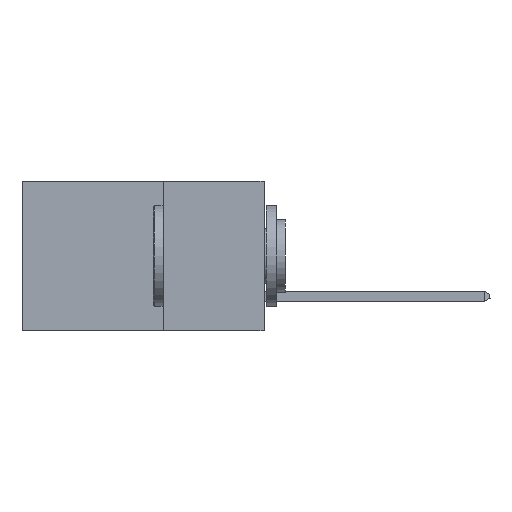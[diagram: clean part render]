
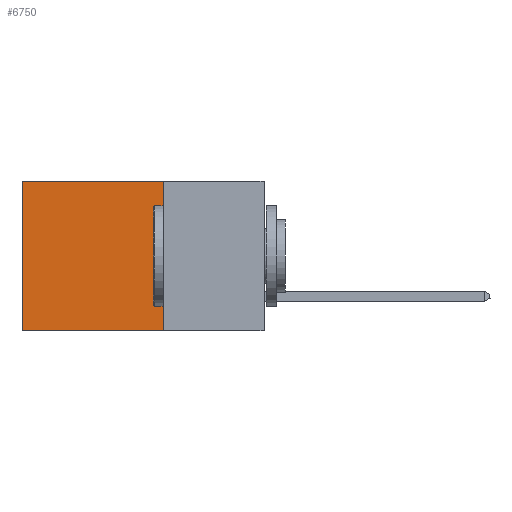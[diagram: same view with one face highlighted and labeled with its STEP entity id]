
A CAD part, left-side view. The second image highlights one B-rep face of the part: STEP entity #6750.
In plain terms, the highlighted planar face has unit normal (-1, 0, 0).
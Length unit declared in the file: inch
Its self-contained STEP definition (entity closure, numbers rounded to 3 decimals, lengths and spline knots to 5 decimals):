
#143 = VERTEX_POINT ( 'NONE', #7188 ) ;
#413 = CARTESIAN_POINT ( 'NONE',  ( 0.298, 0.6, 0. ) ) ;
#593 = LINE ( 'NONE', #413, #1870 ) ;
#605 = VERTEX_POINT ( 'NONE', #2450 ) ;
#1080 = VECTOR ( 'NONE', #4341, 39.37008 ) ;
#1273 = DIRECTION ( 'NONE',  ( 0., 0., -1. ) ) ;
#1441 = VECTOR ( 'NONE', #8896, 39.37008 ) ;
#1870 = VECTOR ( 'NONE', #4337, 39.37008 ) ;
#2033 = CARTESIAN_POINT ( 'NONE',  ( 0.298, 0.25, 0. ) ) ;
#2450 = CARTESIAN_POINT ( 'NONE',  ( 0.298, 0.6, -0.37 ) ) ;
#2784 = CARTESIAN_POINT ( 'NONE',  ( 0.298, 0.25, 0. ) ) ;
#2897 = EDGE_CURVE ( 'NONE', #7381, #605, #6038, .T. ) ;
#3530 = FACE_OUTER_BOUND ( 'NONE', #5600, .T. ) ;
#4065 = VECTOR ( 'NONE', #9885, 39.37008 ) ;
#4132 = LINE ( 'NONE', #2784, #1080 ) ;
#4238 = ORIENTED_EDGE ( 'NONE', *, *, #6983, .T. ) ;
#4337 = DIRECTION ( 'NONE',  ( 0., 0., -1. ) ) ;
#4341 = DIRECTION ( 'NONE',  ( 0., 0., -1. ) ) ;
#5512 = AXIS2_PLACEMENT_3D ( 'NONE', #2033, #9295, #1273 ) ;
#5600 = EDGE_LOOP ( 'NONE', ( #4238, #9982, #10278, #7009 ) ) ;
#6038 = LINE ( 'NONE', #9823, #4065 ) ;
#6285 = CARTESIAN_POINT ( 'NONE',  ( 0.298, 0.25, -0.37 ) ) ;
#6750 = ADVANCED_FACE ( 'NONE', ( #3530 ), #7618, .F. ) ;
#6983 = EDGE_CURVE ( 'NONE', #9833, #605, #593, .T. ) ;
#7009 = ORIENTED_EDGE ( 'NONE', *, *, #8475, .T. ) ;
#7188 = CARTESIAN_POINT ( 'NONE',  ( 0.298, 0.25, 0. ) ) ;
#7381 = VERTEX_POINT ( 'NONE', #6285 ) ;
#7394 = CARTESIAN_POINT ( 'NONE',  ( 0.298, 0.25, 0. ) ) ;
#7618 = PLANE ( 'NONE',  #5512 ) ;
#7889 = EDGE_CURVE ( 'NONE', #143, #7381, #4132, .T. ) ;
#8475 = EDGE_CURVE ( 'NONE', #143, #9833, #8865, .T. ) ;
#8865 = LINE ( 'NONE', #7394, #1441 ) ;
#8896 = DIRECTION ( 'NONE',  ( 0., 1., 0. ) ) ;
#9295 = DIRECTION ( 'NONE',  ( 1., 0., 0. ) ) ;
#9823 = CARTESIAN_POINT ( 'NONE',  ( 0.298, 0.25, -0.37 ) ) ;
#9833 = VERTEX_POINT ( 'NONE', #10358 ) ;
#9885 = DIRECTION ( 'NONE',  ( 0., 1., 0. ) ) ;
#9982 = ORIENTED_EDGE ( 'NONE', *, *, #2897, .F. ) ;
#10278 = ORIENTED_EDGE ( 'NONE', *, *, #7889, .F. ) ;
#10358 = CARTESIAN_POINT ( 'NONE',  ( 0.298, 0.6, 0. ) ) ;
